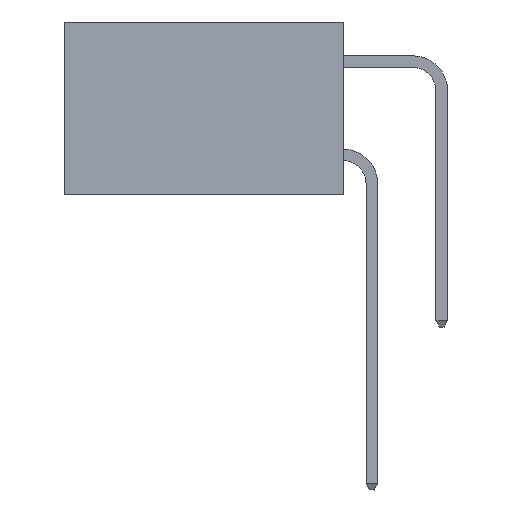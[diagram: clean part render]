
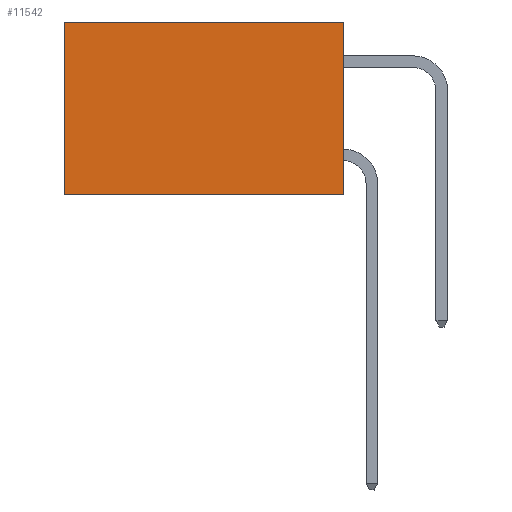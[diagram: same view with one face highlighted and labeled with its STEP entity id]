
A CAD part, left-side view. The second image highlights one B-rep face of the part: STEP entity #11542.
In plain terms, the highlighted planar face has unit normal (-1, 0, 0).
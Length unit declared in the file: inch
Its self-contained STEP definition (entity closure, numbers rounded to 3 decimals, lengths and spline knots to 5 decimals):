
#1390 = EDGE_CURVE ( 'NONE', #14879, #16020, #14194, .T. ) ;
#1436 = VECTOR ( 'NONE', #13427, 39.37008 ) ;
#1772 = VERTEX_POINT ( 'NONE', #15303 ) ;
#2036 = ORIENTED_EDGE ( 'NONE', *, *, #10674, .T. ) ;
#2304 = LINE ( 'NONE', #18688, #10301 ) ;
#2409 = CARTESIAN_POINT ( 'NONE',  ( 0.298, 0.6, 0. ) ) ;
#2899 = VERTEX_POINT ( 'NONE', #2409 ) ;
#3076 = EDGE_CURVE ( 'NONE', #2899, #1772, #12558, .T. ) ;
#4956 = ORIENTED_EDGE ( 'NONE', *, *, #3076, .T. ) ;
#5095 = DIRECTION ( 'NONE',  ( 0., 1., 0. ) ) ;
#5108 = CARTESIAN_POINT ( 'NONE',  ( 0.298, 0., 0. ) ) ;
#5113 = CARTESIAN_POINT ( 'NONE',  ( 0.298, 0., 0. ) ) ;
#5967 = EDGE_LOOP ( 'NONE', ( #4956, #13825, #15821, #2036 ) ) ;
#8076 = FACE_OUTER_BOUND ( 'NONE', #5967, .T. ) ;
#8115 = LINE ( 'NONE', #5113, #16163 ) ;
#8838 = CARTESIAN_POINT ( 'NONE',  ( 0.298, 0., 0. ) ) ;
#9606 = CARTESIAN_POINT ( 'NONE',  ( 0.298, 0., 0. ) ) ;
#10301 = VECTOR ( 'NONE', #20216, 39.37008 ) ;
#10674 = EDGE_CURVE ( 'NONE', #14879, #2899, #8115, .T. ) ;
#11542 = ADVANCED_FACE ( 'NONE', ( #8076 ), #13599, .F. ) ;
#12352 = EDGE_CURVE ( 'NONE', #16020, #1772, #2304, .T. ) ;
#12558 = LINE ( 'NONE', #20264, #17331 ) ;
#13427 = DIRECTION ( 'NONE',  ( 0., 0., -1. ) ) ;
#13599 = PLANE ( 'NONE',  #14364 ) ;
#13825 = ORIENTED_EDGE ( 'NONE', *, *, #12352, .F. ) ;
#14194 = LINE ( 'NONE', #9606, #1436 ) ;
#14364 = AXIS2_PLACEMENT_3D ( 'NONE', #5108, #17685, #17921 ) ;
#14879 = VERTEX_POINT ( 'NONE', #8838 ) ;
#15245 = CARTESIAN_POINT ( 'NONE',  ( 0.298, 0., -0.37 ) ) ;
#15303 = CARTESIAN_POINT ( 'NONE',  ( 0.298, 0.6, -0.37 ) ) ;
#15821 = ORIENTED_EDGE ( 'NONE', *, *, #1390, .F. ) ;
#16020 = VERTEX_POINT ( 'NONE', #15245 ) ;
#16163 = VECTOR ( 'NONE', #5095, 39.37008 ) ;
#17293 = DIRECTION ( 'NONE',  ( 0., 0., -1. ) ) ;
#17331 = VECTOR ( 'NONE', #17293, 39.37008 ) ;
#17685 = DIRECTION ( 'NONE',  ( 1., 0., 0. ) ) ;
#17921 = DIRECTION ( 'NONE',  ( 0., 0., -1. ) ) ;
#18688 = CARTESIAN_POINT ( 'NONE',  ( 0.298, 0., -0.37 ) ) ;
#20216 = DIRECTION ( 'NONE',  ( 0., 1., 0. ) ) ;
#20264 = CARTESIAN_POINT ( 'NONE',  ( 0.298, 0.6, 0. ) ) ;
